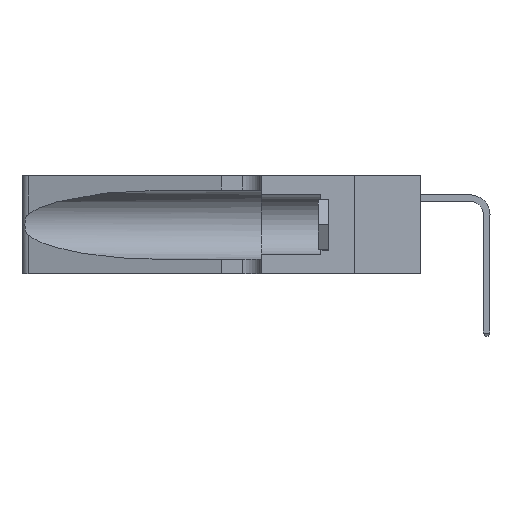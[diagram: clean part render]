
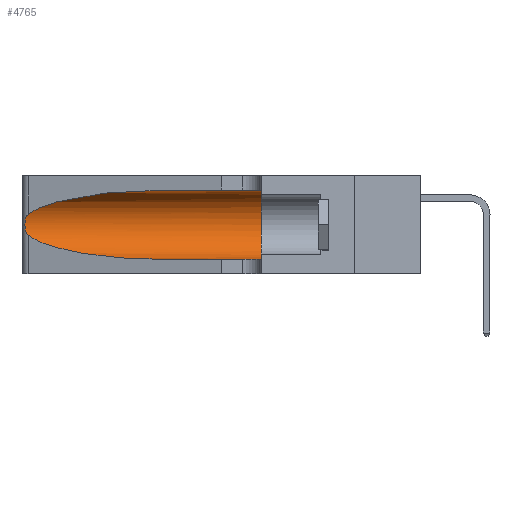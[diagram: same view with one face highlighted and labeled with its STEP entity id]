
A CAD part, left-side view. The second image highlights one B-rep face of the part: STEP entity #4765.
In plain terms, the highlighted cylindrical face has radius 3.308 mm (diameter 6.617 mm), a partial arc.
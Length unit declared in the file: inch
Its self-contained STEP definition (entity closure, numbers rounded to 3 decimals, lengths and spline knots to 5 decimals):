
#231 = DIRECTION ( 'NONE',  ( 0., -1., 0. ) ) ;
#247 = DIRECTION ( 'NONE',  ( 0., -1., 0. ) ) ;
#378 = VERTEX_POINT ( 'NONE', #8536 ) ;
#508 =( BOUNDED_CURVE ( )  B_SPLINE_CURVE ( 3, ( #21939, #8783, #16377, #4985 ),
 .UNSPECIFIED., .F., .T. ) 
 B_SPLINE_CURVE_WITH_KNOTS ( ( 4, 4 ),
 ( 3.44316, 4.71239 ),
 .UNSPECIFIED. ) 
 CURVE ( )  GEOMETRIC_REPRESENTATION_ITEM ( )  RATIONAL_B_SPLINE_CURVE ( ( 1., 0.87, 0.87, 1. ) ) 
 REPRESENTATION_ITEM ( '' )  );
#941 = FACE_OUTER_BOUND ( 'NONE', #10561, .T. ) ;
#1234 = ORIENTED_EDGE ( 'NONE', *, *, #13965, .T. ) ;
#1238 = CARTESIAN_POINT ( 'NONE',  ( 0.2373, 1.15595, 0.28018 ) ) ;
#1319 = CARTESIAN_POINT ( 'NONE',  ( 0.25487, 1.22718, 0.22369 ) ) ;
#1452 = EDGE_CURVE ( 'NONE', #15505, #21704, #14911, .T. ) ;
#1998 = VECTOR ( 'NONE', #247, 39.37008 ) ;
#2443 = CARTESIAN_POINT ( 'NONE',  ( 0.25787, 1.23484, 0.2124 ) ) ;
#4368 = CARTESIAN_POINT ( 'NONE',  ( 0.25487, 1.22718, 0.14631 ) ) ;
#4374 = CARTESIAN_POINT ( 'NONE',  ( 0.26018, 1.23835, 0.19895 ) ) ;
#4670 = ORIENTED_EDGE ( 'NONE', *, *, #19236, .F. ) ;
#4765 = ADVANCED_FACE ( 'NONE', ( #941 ), #20036, .F. ) ;
#4818 = VERTEX_POINT ( 'NONE', #4368 ) ;
#4985 = CARTESIAN_POINT ( 'NONE',  ( 0.1305, 0.72297, 0.05475 ) ) ;
#5094 = EDGE_CURVE ( 'NONE', #5560, #24523, #5367, .T. ) ;
#5367 =( BOUNDED_CURVE ( )  B_SPLINE_CURVE ( 3, ( #12838, #14634, #1238, #1319 ),
 .UNSPECIFIED., .F., .T. ) 
 B_SPLINE_CURVE_WITH_KNOTS ( ( 4, 4 ),
 ( 1.5708, 2.84003 ),
 .UNSPECIFIED. ) 
 CURVE ( )  GEOMETRIC_REPRESENTATION_ITEM ( )  RATIONAL_B_SPLINE_CURVE ( ( 1., 0.87, 0.87, 1. ) ) 
 REPRESENTATION_ITEM ( '' )  );
#5560 = VERTEX_POINT ( 'NONE', #23579 ) ;
#6314 = CARTESIAN_POINT ( 'NONE',  ( 0.26075, 1.23896, 0.178 ) ) ;
#6522 = LINE ( 'NONE', #22986, #1998 ) ;
#7943 = CARTESIAN_POINT ( 'NONE',  ( 0.25487, 1.22718, 0.22369 ) ) ;
#8242 = B_SPLINE_CURVE_WITH_KNOTS ( 'NONE', 3,
 ( #21350, #17516, #13895, #2443, #15788, #4374, #17687, #6314, #19581, #8259, #21431, #10164, #23285, #12094 ),
 .UNSPECIFIED., .F., .F.,
 ( 4, 2, 2, 2, 2, 2, 4 ),
 ( 0., 0.00027, 0.00053, 0.00107, 0.0016, 0.00187, 0.00214 ),
 .UNSPECIFIED. ) ;
#8259 = CARTESIAN_POINT ( 'NONE',  ( 0.25856, 1.23593, 0.16098 ) ) ;
#8396 = CARTESIAN_POINT ( 'NONE',  ( 0.1305, 0.35, 0.31525 ) ) ;
#8536 = CARTESIAN_POINT ( 'NONE',  ( 0.1305, 0.72297, 0.05475 ) ) ;
#8783 = CARTESIAN_POINT ( 'NONE',  ( 0.2373, 1.15595, 0.08982 ) ) ;
#9785 = ORIENTED_EDGE ( 'NONE', *, *, #5094, .T. ) ;
#9836 = CARTESIAN_POINT ( 'NONE',  ( 0.1305, 1.61858, 0.185 ) ) ;
#9966 = CARTESIAN_POINT ( 'NONE',  ( 0.1305, 0.35, 0.185 ) ) ;
#10164 = CARTESIAN_POINT ( 'NONE',  ( 0.25639, 1.23186, 0.15144 ) ) ;
#10448 = ORIENTED_EDGE ( 'NONE', *, *, #1452, .F. ) ;
#10561 = EDGE_LOOP ( 'NONE', ( #9785, #17130, #1234, #21731, #10448, #4670 ) ) ;
#11899 = DIRECTION ( 'NONE',  ( 0., 0., 1. ) ) ;
#12094 = CARTESIAN_POINT ( 'NONE',  ( 0.25487, 1.22718, 0.14631 ) ) ;
#12838 = CARTESIAN_POINT ( 'NONE',  ( 0.1305, 0.72297, 0.31525 ) ) ;
#13895 = CARTESIAN_POINT ( 'NONE',  ( 0.25639, 1.23184, 0.21858 ) ) ;
#13965 = EDGE_CURVE ( 'NONE', #4818, #378, #508, .T. ) ;
#14634 = CARTESIAN_POINT ( 'NONE',  ( 0.18966, 0.96281, 0.31525 ) ) ;
#14782 = EDGE_CURVE ( 'NONE', #24523, #4818, #8242, .T. ) ;
#14911 = CIRCLE ( 'NONE', #23561, 0.13025 ) ;
#15505 = VERTEX_POINT ( 'NONE', #8396 ) ;
#15788 = CARTESIAN_POINT ( 'NONE',  ( 0.25854, 1.2359, 0.20912 ) ) ;
#16377 = CARTESIAN_POINT ( 'NONE',  ( 0.18966, 0.96281, 0.05475 ) ) ;
#17130 = ORIENTED_EDGE ( 'NONE', *, *, #14782, .T. ) ;
#17304 = CARTESIAN_POINT ( 'NONE',  ( 0.1305, 1.61858, 0.31525 ) ) ;
#17436 = DIRECTION ( 'NONE',  ( 0., 0., -1. ) ) ;
#17516 = CARTESIAN_POINT ( 'NONE',  ( 0.25555, 1.22994, 0.2215 ) ) ;
#17687 = CARTESIAN_POINT ( 'NONE',  ( 0.26075, 1.23896, 0.19203 ) ) ;
#19220 = DIRECTION ( 'NONE',  ( 0., -1., 0. ) ) ;
#19236 = EDGE_CURVE ( 'NONE', #5560, #15505, #19830, .T. ) ;
#19239 = VECTOR ( 'NONE', #19220, 39.37008 ) ;
#19581 = CARTESIAN_POINT ( 'NONE',  ( 0.26017, 1.23833, 0.17102 ) ) ;
#19830 = LINE ( 'NONE', #17304, #19239 ) ;
#20036 = CYLINDRICAL_SURFACE ( 'NONE', #22673, 0.13025 ) ;
#21350 = CARTESIAN_POINT ( 'NONE',  ( 0.25487, 1.22718, 0.22369 ) ) ;
#21431 = CARTESIAN_POINT ( 'NONE',  ( 0.25789, 1.23486, 0.15765 ) ) ;
#21704 = VERTEX_POINT ( 'NONE', #21918 ) ;
#21731 = ORIENTED_EDGE ( 'NONE', *, *, #24522, .T. ) ;
#21918 = CARTESIAN_POINT ( 'NONE',  ( 0.1305, 0.35, 0.05475 ) ) ;
#21939 = CARTESIAN_POINT ( 'NONE',  ( 0.25487, 1.22718, 0.14631 ) ) ;
#22673 = AXIS2_PLACEMENT_3D ( 'NONE', #9836, #231, #17436 ) ;
#22986 = CARTESIAN_POINT ( 'NONE',  ( 0.1305, 1.61858, 0.05475 ) ) ;
#23092 = DIRECTION ( 'NONE',  ( 0., 1., 0. ) ) ;
#23285 = CARTESIAN_POINT ( 'NONE',  ( 0.25555, 1.22993, 0.14849 ) ) ;
#23561 = AXIS2_PLACEMENT_3D ( 'NONE', #9966, #23092, #11899 ) ;
#23579 = CARTESIAN_POINT ( 'NONE',  ( 0.1305, 0.72297, 0.31525 ) ) ;
#24522 = EDGE_CURVE ( 'NONE', #378, #21704, #6522, .T. ) ;
#24523 = VERTEX_POINT ( 'NONE', #7943 ) ;
